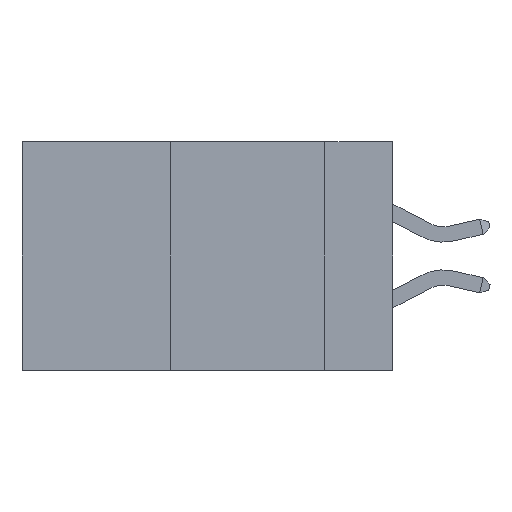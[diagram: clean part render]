
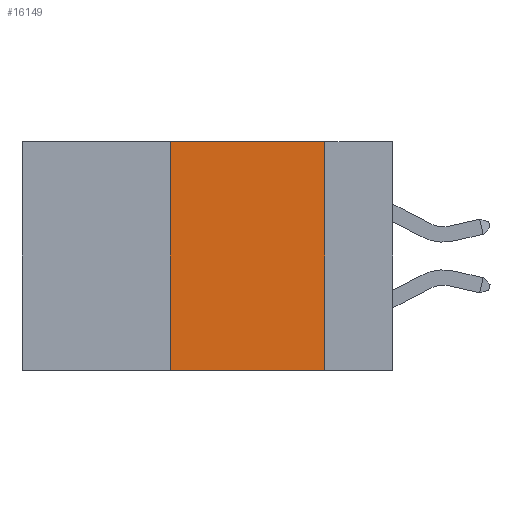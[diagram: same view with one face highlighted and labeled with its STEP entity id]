
A CAD part, left-side view. The second image highlights one B-rep face of the part: STEP entity #16149.
In plain terms, the highlighted planar face has unit normal (-1, 0, 0).
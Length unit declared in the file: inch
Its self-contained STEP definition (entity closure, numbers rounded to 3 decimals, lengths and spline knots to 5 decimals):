
#222 = AXIS2_PLACEMENT_3D ( 'NONE', #14058, #3152, #1108 ) ;
#377 = VERTEX_POINT ( 'NONE', #17607 ) ;
#524 = DIRECTION ( 'NONE',  ( 0., 0., 1. ) ) ;
#1108 = DIRECTION ( 'NONE',  ( 0., 0., -1. ) ) ;
#1542 = LINE ( 'NONE', #1573, #5923 ) ;
#1573 = CARTESIAN_POINT ( 'NONE',  ( 0., 0.6, -0.37 ) ) ;
#1589 = VECTOR ( 'NONE', #524, 39.37008 ) ;
#3152 = DIRECTION ( 'NONE',  ( 1., 0., 0. ) ) ;
#3433 = PLANE ( 'NONE',  #222 ) ;
#3877 = EDGE_CURVE ( 'NONE', #23362, #377, #8422, .T. ) ;
#4608 = VERTEX_POINT ( 'NONE', #21469 ) ;
#5923 = VECTOR ( 'NONE', #16768, 39.37008 ) ;
#5970 = ORIENTED_EDGE ( 'NONE', *, *, #16502, .F. ) ;
#6909 = DIRECTION ( 'NONE',  ( 0., 0., -1. ) ) ;
#7015 = FACE_OUTER_BOUND ( 'NONE', #12121, .T. ) ;
#7971 = EDGE_CURVE ( 'NONE', #377, #19213, #17288, .T. ) ;
#8422 = LINE ( 'NONE', #21157, #17261 ) ;
#11078 = CARTESIAN_POINT ( 'NONE',  ( 0., 0.36, 0. ) ) ;
#11167 = EDGE_CURVE ( 'NONE', #4608, #19213, #1542, .T. ) ;
#12068 = ORIENTED_EDGE ( 'NONE', *, *, #3877, .F. ) ;
#12121 = EDGE_LOOP ( 'NONE', ( #16601, #12068, #5970, #22399 ) ) ;
#13729 = CARTESIAN_POINT ( 'NONE',  ( 0., 0.11, 0. ) ) ;
#13913 = CARTESIAN_POINT ( 'NONE',  ( 0., 0.11, -0.37 ) ) ;
#14058 = CARTESIAN_POINT ( 'NONE',  ( 0., 0.6, 0. ) ) ;
#14828 = LINE ( 'NONE', #11078, #1589 ) ;
#14894 = VECTOR ( 'NONE', #6909, 39.37008 ) ;
#16149 = ADVANCED_FACE ( 'NONE', ( #7015 ), #3433, .F. ) ;
#16502 = EDGE_CURVE ( 'NONE', #4608, #23362, #14828, .T. ) ;
#16601 = ORIENTED_EDGE ( 'NONE', *, *, #7971, .F. ) ;
#16768 = DIRECTION ( 'NONE',  ( 0., -1., 0. ) ) ;
#17261 = VECTOR ( 'NONE', #18675, 39.37008 ) ;
#17288 = LINE ( 'NONE', #13729, #14894 ) ;
#17607 = CARTESIAN_POINT ( 'NONE',  ( 0., 0.11, 0. ) ) ;
#18675 = DIRECTION ( 'NONE',  ( 0., -1., 0. ) ) ;
#19213 = VERTEX_POINT ( 'NONE', #13913 ) ;
#21157 = CARTESIAN_POINT ( 'NONE',  ( 0., 0.6, 0. ) ) ;
#21469 = CARTESIAN_POINT ( 'NONE',  ( 0., 0.36, -0.37 ) ) ;
#22399 = ORIENTED_EDGE ( 'NONE', *, *, #11167, .T. ) ;
#23362 = VERTEX_POINT ( 'NONE', #24117 ) ;
#24117 = CARTESIAN_POINT ( 'NONE',  ( 0., 0.36, 0. ) ) ;
